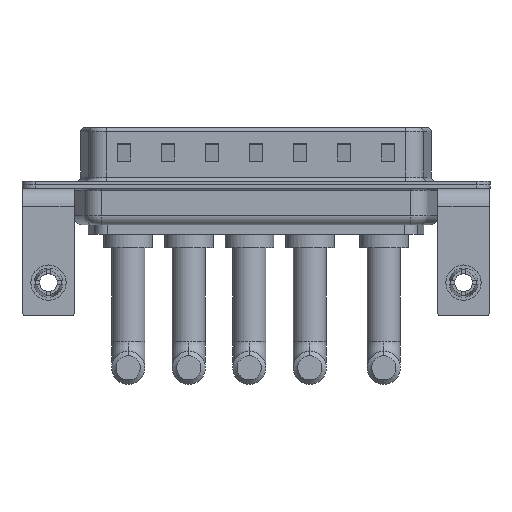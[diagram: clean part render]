
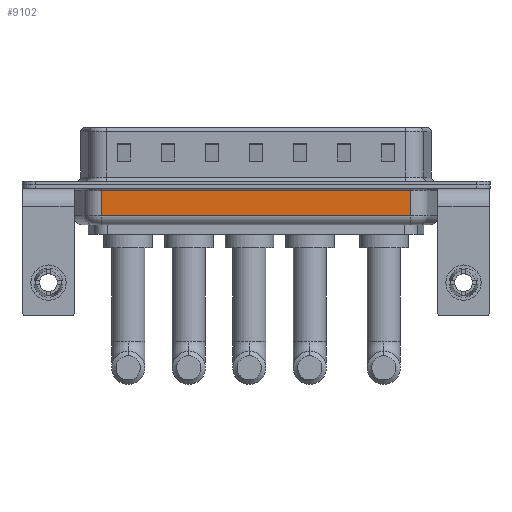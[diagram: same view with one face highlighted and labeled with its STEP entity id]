
A CAD part, front view. The second image highlights one B-rep face of the part: STEP entity #9102.
In plain terms, the highlighted planar face has unit normal (0, -1, 0).
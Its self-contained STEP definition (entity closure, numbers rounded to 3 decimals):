
#169 = ORIENTED_EDGE ( 'NONE', *, *, #8314, .T. ) ;
#780 = ORIENTED_EDGE ( 'NONE', *, *, #14318, .F. ) ;
#1147 = DIRECTION ( 'NONE',  ( 0., 0., 1. ) ) ;
#1176 = EDGE_CURVE ( 'NONE', #11485, #16273, #15356, .T. ) ;
#1605 = VECTOR ( 'NONE', #13890, 1000. ) ;
#2187 = LINE ( 'NONE', #12792, #2851 ) ;
#2851 = VECTOR ( 'NONE', #1147, 1000. ) ;
#3028 = CARTESIAN_POINT ( 'NONE',  ( 41.044, -5.35, -0.65 ) ) ;
#3698 = AXIS2_PLACEMENT_3D ( 'NONE', #4773, #10883, #16107 ) ;
#3799 = CARTESIAN_POINT ( 'NONE',  ( 6.006, -5.35, -3.5 ) ) ;
#4301 = VERTEX_POINT ( 'NONE', #10046 ) ;
#4344 = VECTOR ( 'NONE', #12879, 1000. ) ;
#4773 = CARTESIAN_POINT ( 'NONE',  ( 6.006, -5.35, -4.5 ) ) ;
#4870 = CARTESIAN_POINT ( 'NONE',  ( 6.006, -5.35, -3.5 ) ) ;
#5090 = EDGE_CURVE ( 'NONE', #9778, #4301, #12164, .T. ) ;
#5410 = DIRECTION ( 'NONE',  ( -1., 0., 0. ) ) ;
#6195 = LINE ( 'NONE', #6283, #4344 ) ;
#6283 = CARTESIAN_POINT ( 'NONE',  ( 6.006, -5.35, -4.5 ) ) ;
#8314 = EDGE_CURVE ( 'NONE', #16273, #9778, #2187, .T. ) ;
#9102 = ADVANCED_FACE ( 'NONE', ( #14816 ), #13927, .F. ) ;
#9778 = VERTEX_POINT ( 'NONE', #3028 ) ;
#9923 = ORIENTED_EDGE ( 'NONE', *, *, #5090, .T. ) ;
#10046 = CARTESIAN_POINT ( 'NONE',  ( 6.006, -5.35, -0.65 ) ) ;
#10883 = DIRECTION ( 'NONE',  ( 0., 1., 0. ) ) ;
#11485 = VERTEX_POINT ( 'NONE', #4870 ) ;
#11915 = CARTESIAN_POINT ( 'NONE',  ( 6.006, -5.35, -0.65 ) ) ;
#12164 = LINE ( 'NONE', #11915, #14710 ) ;
#12792 = CARTESIAN_POINT ( 'NONE',  ( 41.044, -5.35, -4.5 ) ) ;
#12879 = DIRECTION ( 'NONE',  ( 0., 0., 1. ) ) ;
#13735 = ORIENTED_EDGE ( 'NONE', *, *, #1176, .T. ) ;
#13890 = DIRECTION ( 'NONE',  ( 1., 0., 0. ) ) ;
#13927 = PLANE ( 'NONE',  #3698 ) ;
#14318 = EDGE_CURVE ( 'NONE', #11485, #4301, #6195, .T. ) ;
#14710 = VECTOR ( 'NONE', #5410, 1000. ) ;
#14816 = FACE_OUTER_BOUND ( 'NONE', #16947, .T. ) ;
#15148 = CARTESIAN_POINT ( 'NONE',  ( 41.044, -5.35, -3.5 ) ) ;
#15356 = LINE ( 'NONE', #3799, #1605 ) ;
#16107 = DIRECTION ( 'NONE',  ( 0., 0., 1. ) ) ;
#16273 = VERTEX_POINT ( 'NONE', #15148 ) ;
#16947 = EDGE_LOOP ( 'NONE', ( #780, #13735, #169, #9923 ) ) ;
